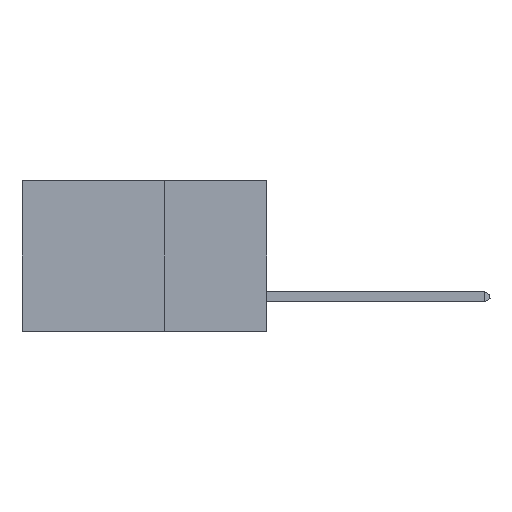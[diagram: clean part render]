
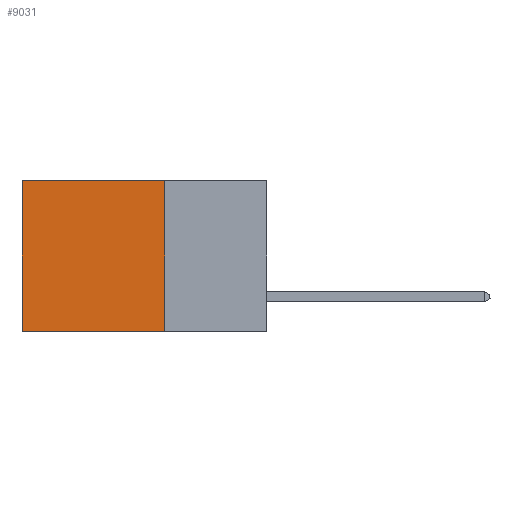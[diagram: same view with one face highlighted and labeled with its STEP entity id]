
A CAD part, left-side view. The second image highlights one B-rep face of the part: STEP entity #9031.
In plain terms, the highlighted planar face has unit normal (-1, 0, 0).
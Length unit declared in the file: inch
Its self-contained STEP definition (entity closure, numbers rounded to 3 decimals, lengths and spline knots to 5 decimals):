
#379 = CARTESIAN_POINT ( 'NONE',  ( 0.2875, 0.6, 0. ) ) ;
#1601 = DIRECTION ( 'NONE',  ( 1., 0., 0. ) ) ;
#1689 = LINE ( 'NONE', #5564, #4680 ) ;
#3179 = EDGE_CURVE ( 'NONE', #16163, #7755, #1689, .T. ) ;
#3401 = VECTOR ( 'NONE', #13941, 39.37008 ) ;
#3693 = DIRECTION ( 'NONE',  ( 0., 1., 0. ) ) ;
#4094 = VERTEX_POINT ( 'NONE', #6724 ) ;
#4188 = DIRECTION ( 'NONE',  ( 0., 0., -1. ) ) ;
#4248 = DIRECTION ( 'NONE',  ( 0., 0., -1. ) ) ;
#4680 = VECTOR ( 'NONE', #3693, 39.37008 ) ;
#5461 = PLANE ( 'NONE',  #7013 ) ;
#5530 = EDGE_LOOP ( 'NONE', ( #9324, #13651, #21202, #5857 ) ) ;
#5564 = CARTESIAN_POINT ( 'NONE',  ( 0.2875, 0.25, -0.37 ) ) ;
#5857 = ORIENTED_EDGE ( 'NONE', *, *, #21518, .T. ) ;
#5927 = EDGE_CURVE ( 'NONE', #4094, #16163, #6016, .T. ) ;
#6016 = LINE ( 'NONE', #23537, #12308 ) ;
#6368 = EDGE_CURVE ( 'NONE', #7767, #7755, #18008, .T. ) ;
#6724 = CARTESIAN_POINT ( 'NONE',  ( 0.2875, 0.25, 0. ) ) ;
#7013 = AXIS2_PLACEMENT_3D ( 'NONE', #24537, #1601, #17002 ) ;
#7755 = VERTEX_POINT ( 'NONE', #21836 ) ;
#7767 = VERTEX_POINT ( 'NONE', #9926 ) ;
#9031 = ADVANCED_FACE ( 'NONE', ( #22813 ), #5461, .F. ) ;
#9324 = ORIENTED_EDGE ( 'NONE', *, *, #6368, .T. ) ;
#9926 = CARTESIAN_POINT ( 'NONE',  ( 0.2875, 0.6, 0. ) ) ;
#12308 = VECTOR ( 'NONE', #4188, 39.37008 ) ;
#13651 = ORIENTED_EDGE ( 'NONE', *, *, #3179, .F. ) ;
#13941 = DIRECTION ( 'NONE',  ( 0., 1., 0. ) ) ;
#15664 = LINE ( 'NONE', #23102, #3401 ) ;
#16163 = VERTEX_POINT ( 'NONE', #17821 ) ;
#17002 = DIRECTION ( 'NONE',  ( 0., 0., -1. ) ) ;
#17821 = CARTESIAN_POINT ( 'NONE',  ( 0.2875, 0.25, -0.37 ) ) ;
#18008 = LINE ( 'NONE', #379, #24268 ) ;
#21202 = ORIENTED_EDGE ( 'NONE', *, *, #5927, .F. ) ;
#21518 = EDGE_CURVE ( 'NONE', #4094, #7767, #15664, .T. ) ;
#21836 = CARTESIAN_POINT ( 'NONE',  ( 0.2875, 0.6, -0.37 ) ) ;
#22813 = FACE_OUTER_BOUND ( 'NONE', #5530, .T. ) ;
#23102 = CARTESIAN_POINT ( 'NONE',  ( 0.2875, 0.25, 0. ) ) ;
#23537 = CARTESIAN_POINT ( 'NONE',  ( 0.2875, 0.25, 0. ) ) ;
#24268 = VECTOR ( 'NONE', #4248, 39.37008 ) ;
#24537 = CARTESIAN_POINT ( 'NONE',  ( 0.2875, 0.25, 0. ) ) ;
